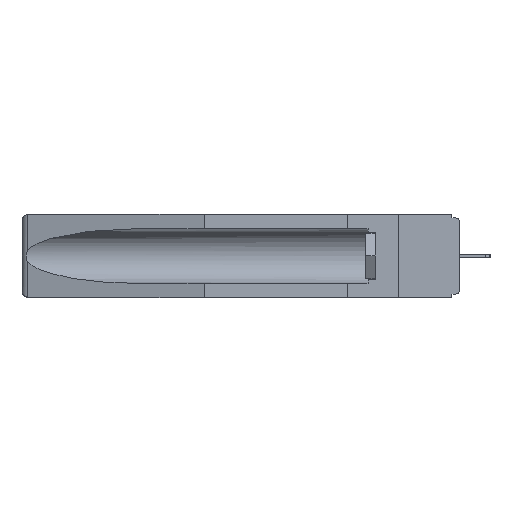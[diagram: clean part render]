
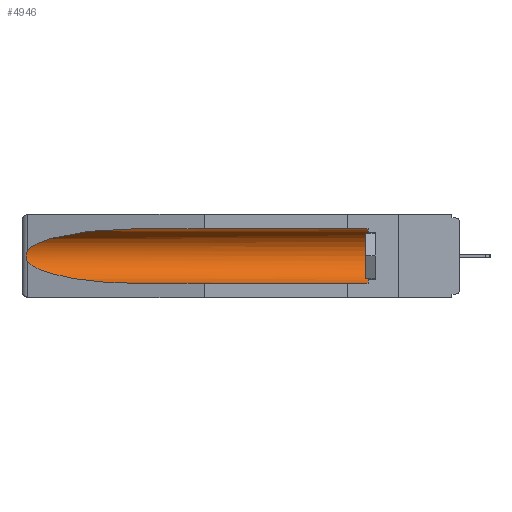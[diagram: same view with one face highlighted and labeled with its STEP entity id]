
A CAD part, left-side view. The second image highlights one B-rep face of the part: STEP entity #4946.
In plain terms, the highlighted cylindrical face has radius 2.857 mm (diameter 5.715 mm), a partial arc.
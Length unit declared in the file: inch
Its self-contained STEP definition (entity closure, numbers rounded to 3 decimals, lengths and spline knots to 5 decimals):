
#662 =( BOUNDED_CURVE ( )  B_SPLINE_CURVE ( 3, ( #21950, #22035, #28596, #8765 ),
 .UNSPECIFIED., .F., .F. ) 
 B_SPLINE_CURVE_WITH_KNOTS ( ( 4, 4 ),
 ( 0.1948, 1.5708 ),
 .UNSPECIFIED. ) 
 CURVE ( )  GEOMETRIC_REPRESENTATION_ITEM ( )  RATIONAL_B_SPLINE_CURVE ( ( 1., 0.848, 0.848, 1. ) ) 
 REPRESENTATION_ITEM ( '' )  );
#1406 = CARTESIAN_POINT ( 'NONE',  ( 0.26655, 1.53094, -0.18657 ) ) ;
#1439 = DIRECTION ( 'NONE',  ( 0., -1., 0. ) ) ;
#1543 = EDGE_LOOP ( 'NONE', ( #21432, #14012, #23538, #14306, #17261, #24598 ) ) ;
#1745 = DIRECTION ( 'NONE',  ( 0., 0., 1. ) ) ;
#1774 = CARTESIAN_POINT ( 'NONE',  ( 0.26537, 1.52718, -0.14972 ) ) ;
#2550 = CARTESIAN_POINT ( 'NONE',  ( 0.26537, 1.52718, -0.14972 ) ) ;
#3977 = VECTOR ( 'NONE', #16929, 39.37008 ) ;
#4226 = AXIS2_PLACEMENT_3D ( 'NONE', #23627, #1439, #21223 ) ;
#4699 = VECTOR ( 'NONE', #13056, 39.37008 ) ;
#4708 = VERTEX_POINT ( 'NONE', #20127 ) ;
#4946 = ADVANCED_FACE ( 'NONE', ( #26184 ), #14398, .F. ) ;
#5837 = CARTESIAN_POINT ( 'NONE',  ( 0.2673, 1.5327, -0.16383 ) ) ;
#5931 = CARTESIAN_POINT ( 'NONE',  ( 0.26654, 1.53092, -0.15636 ) ) ;
#6542 = VERTEX_POINT ( 'NONE', #12035 ) ;
#8065 = CARTESIAN_POINT ( 'NONE',  ( 0.26597, 1.5296, -0.19026 ) ) ;
#8191 = LINE ( 'NONE', #8489, #4699 ) ;
#8466 = B_SPLINE_CURVE_WITH_KNOTS ( 'NONE', 3,
 ( #2550, #26995, #5931, #5837, #27809, #14584, #21369, #1406, #8065, #28027 ),
 .UNSPECIFIED., .F., .F.,
 ( 4, 2, 2, 2, 4 ),
 ( 0., 0.00029, 0.00058, 0.00087, 0.00117 ),
 .UNSPECIFIED. ) ;
#8489 = CARTESIAN_POINT ( 'NONE',  ( 0.155, -0.30754, -0.284 ) ) ;
#8765 = CARTESIAN_POINT ( 'NONE',  ( 0.155, 1.07973, -0.284 ) ) ;
#9161 = VERTEX_POINT ( 'NONE', #21447 ) ;
#10124 = CARTESIAN_POINT ( 'NONE',  ( 0.155, -0.30754, -0.059 ) ) ;
#10318 = CARTESIAN_POINT ( 'NONE',  ( 0.21114, 1.30732, -0.059 ) ) ;
#10415 = EDGE_CURVE ( 'NONE', #6542, #10853, #8191, .T. ) ;
#10612 =( BOUNDED_CURVE ( )  B_SPLINE_CURVE ( 3, ( #14656, #10318, #14959, #1774 ),
 .UNSPECIFIED., .F., .F. ) 
 B_SPLINE_CURVE_WITH_KNOTS ( ( 4, 4 ),
 ( 4.71239, 6.08839 ),
 .UNSPECIFIED. ) 
 CURVE ( )  GEOMETRIC_REPRESENTATION_ITEM ( )  RATIONAL_B_SPLINE_CURVE ( ( 1., 0.848, 0.848, 1. ) ) 
 REPRESENTATION_ITEM ( '' )  );
#10853 = VERTEX_POINT ( 'NONE', #20065 ) ;
#11108 = EDGE_CURVE ( 'NONE', #13477, #25558, #13721, .T. ) ;
#11974 = CARTESIAN_POINT ( 'NONE',  ( 0.155, 0.126, -0.059 ) ) ;
#12035 = CARTESIAN_POINT ( 'NONE',  ( 0.155, 0.126, -0.284 ) ) ;
#13056 = DIRECTION ( 'NONE',  ( 0., 1., 0. ) ) ;
#13477 = VERTEX_POINT ( 'NONE', #11974 ) ;
#13721 = LINE ( 'NONE', #10124, #3977 ) ;
#14012 = ORIENTED_EDGE ( 'NONE', *, *, #21346, .T. ) ;
#14306 = ORIENTED_EDGE ( 'NONE', *, *, #10415, .F. ) ;
#14398 = CYLINDRICAL_SURFACE ( 'NONE', #21256, 0.1125 ) ;
#14584 = CARTESIAN_POINT ( 'NONE',  ( 0.2675, 1.53308, -0.17534 ) ) ;
#14624 = DIRECTION ( 'NONE',  ( 0., 1., 0. ) ) ;
#14656 = CARTESIAN_POINT ( 'NONE',  ( 0.155, 1.07973, -0.059 ) ) ;
#14959 = CARTESIAN_POINT ( 'NONE',  ( 0.25451, 1.48313, -0.09465 ) ) ;
#16929 = DIRECTION ( 'NONE',  ( 0., 1., 0. ) ) ;
#17073 = CARTESIAN_POINT ( 'NONE',  ( 0.155, -0.30754, -0.1715 ) ) ;
#17261 = ORIENTED_EDGE ( 'NONE', *, *, #20349, .T. ) ;
#19197 = EDGE_CURVE ( 'NONE', #25558, #4708, #10612, .T. ) ;
#20065 = CARTESIAN_POINT ( 'NONE',  ( 0.155, 1.07973, -0.284 ) ) ;
#20127 = CARTESIAN_POINT ( 'NONE',  ( 0.26537, 1.52718, -0.14972 ) ) ;
#20173 = EDGE_CURVE ( 'NONE', #9161, #10853, #662, .T. ) ;
#20349 = EDGE_CURVE ( 'NONE', #6542, #13477, #22717, .T. ) ;
#21223 = DIRECTION ( 'NONE',  ( 0., 0., 1. ) ) ;
#21256 = AXIS2_PLACEMENT_3D ( 'NONE', #17073, #14624, #1745 ) ;
#21346 = EDGE_CURVE ( 'NONE', #4708, #9161, #8466, .T. ) ;
#21369 = CARTESIAN_POINT ( 'NONE',  ( 0.2673, 1.53269, -0.17917 ) ) ;
#21432 = ORIENTED_EDGE ( 'NONE', *, *, #19197, .T. ) ;
#21447 = CARTESIAN_POINT ( 'NONE',  ( 0.26537, 1.52718, -0.19328 ) ) ;
#21950 = CARTESIAN_POINT ( 'NONE',  ( 0.26537, 1.52718, -0.19328 ) ) ;
#22035 = CARTESIAN_POINT ( 'NONE',  ( 0.25451, 1.48313, -0.24835 ) ) ;
#22717 = CIRCLE ( 'NONE', #4226, 0.1125 ) ;
#23538 = ORIENTED_EDGE ( 'NONE', *, *, #20173, .T. ) ;
#23627 = CARTESIAN_POINT ( 'NONE',  ( 0.155, 0.126, -0.1715 ) ) ;
#24002 = CARTESIAN_POINT ( 'NONE',  ( 0.155, 1.07973, -0.059 ) ) ;
#24598 = ORIENTED_EDGE ( 'NONE', *, *, #11108, .T. ) ;
#25558 = VERTEX_POINT ( 'NONE', #24002 ) ;
#26184 = FACE_OUTER_BOUND ( 'NONE', #1543, .T. ) ;
#26995 = CARTESIAN_POINT ( 'NONE',  ( 0.26597, 1.52961, -0.15275 ) ) ;
#27809 = CARTESIAN_POINT ( 'NONE',  ( 0.2675, 1.53308, -0.16763 ) ) ;
#28027 = CARTESIAN_POINT ( 'NONE',  ( 0.26537, 1.52718, -0.19328 ) ) ;
#28596 = CARTESIAN_POINT ( 'NONE',  ( 0.21114, 1.30732, -0.284 ) ) ;
